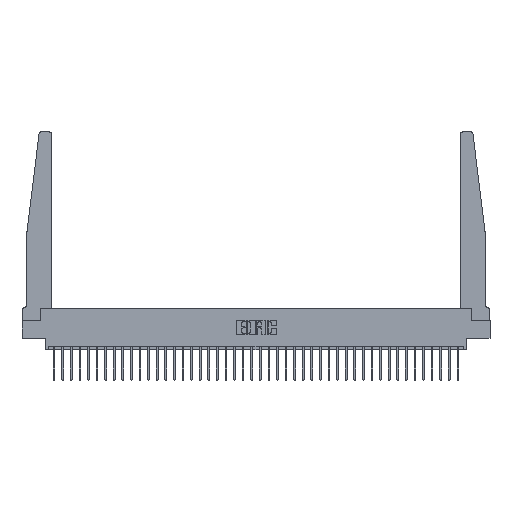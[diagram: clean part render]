
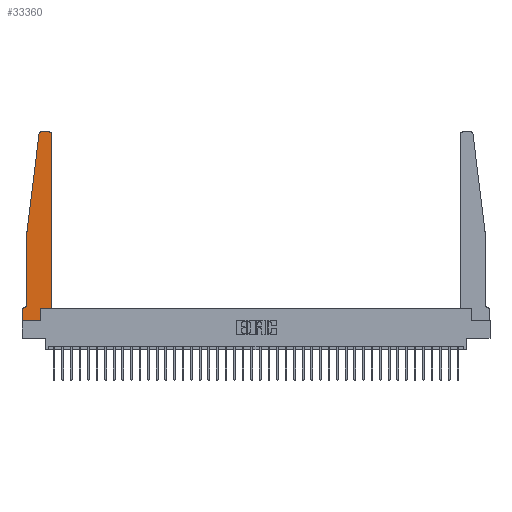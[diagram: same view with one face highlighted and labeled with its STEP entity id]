
A CAD part, top view. The second image highlights one B-rep face of the part: STEP entity #33360.
In plain terms, the highlighted planar face has unit normal (0, 0, 1).
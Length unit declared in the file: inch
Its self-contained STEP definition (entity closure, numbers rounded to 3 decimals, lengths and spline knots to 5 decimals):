
#503 = VECTOR ( 'NONE', #7519, 39.37008 ) ;
#725 = CARTESIAN_POINT ( 'NONE',  ( 0.065, 1.25, 0.37 ) ) ;
#1184 = EDGE_CURVE ( 'NONE', #20355, #28076, #22649, .T. ) ;
#1541 = DIRECTION ( 'NONE',  ( 0., 1., 0. ) ) ;
#1736 = ORIENTED_EDGE ( 'NONE', *, *, #19785, .T. ) ;
#2650 = CARTESIAN_POINT ( 'NONE',  ( 0.2605, 0., 0.37 ) ) ;
#3480 = CARTESIAN_POINT ( 'NONE',  ( 0.2605, 0.18, 0.37 ) ) ;
#3515 = ORIENTED_EDGE ( 'NONE', *, *, #10122, .T. ) ;
#4983 = EDGE_CURVE ( 'NONE', #23676, #20355, #24032, .T. ) ;
#5235 = EDGE_LOOP ( 'NONE', ( #27498, #21151, #14736, #30048, #1736, #3515, #18180, #26234, #5268, #14332, #15177, #31348 ) ) ;
#5259 = CARTESIAN_POINT ( 'NONE',  ( 0.27653, 2.72, 0.37 ) ) ;
#5268 = ORIENTED_EDGE ( 'NONE', *, *, #14583, .T. ) ;
#5748 = VECTOR ( 'NONE', #14102, 39.37008 ) ;
#5788 = LINE ( 'NONE', #28408, #20397 ) ;
#7519 = DIRECTION ( 'NONE',  ( 1., 0., 0. ) ) ;
#8059 = DIRECTION ( 'NONE',  ( 1., 0., 0. ) ) ;
#8507 = VERTEX_POINT ( 'NONE', #22959 ) ;
#8727 = CARTESIAN_POINT ( 'NONE',  ( 0.065, 0.2375, 0.37 ) ) ;
#9334 = DIRECTION ( 'NONE',  ( -1., 0., 0. ) ) ;
#9636 = EDGE_CURVE ( 'NONE', #8507, #23676, #5788, .T. ) ;
#9638 = DIRECTION ( 'NONE',  ( 0., 0., 1. ) ) ;
#9704 = CARTESIAN_POINT ( 'NONE',  ( 0.425, 2.72, 0.37 ) ) ;
#9850 = EDGE_CURVE ( 'NONE', #31163, #11322, #15240, .T. ) ;
#9877 = LINE ( 'NONE', #23579, #30777 ) ;
#10122 = EDGE_CURVE ( 'NONE', #10125, #17348, #14800, .T. ) ;
#10125 = VERTEX_POINT ( 'NONE', #14221 ) ;
#11322 = VERTEX_POINT ( 'NONE', #2650 ) ;
#11602 = DIRECTION ( 'NONE',  ( 0., 0., -1. ) ) ;
#12517 = AXIS2_PLACEMENT_3D ( 'NONE', #27898, #11602, #30634 ) ;
#12874 = DIRECTION ( 'NONE',  ( 0., 0., 1. ) ) ;
#13683 = VECTOR ( 'NONE', #19282, 39.37008 ) ;
#13777 = CARTESIAN_POINT ( 'NONE',  ( 0.2605, 0.18, 0.37 ) ) ;
#14102 = DIRECTION ( 'NONE',  ( -1., 0., 0. ) ) ;
#14221 = CARTESIAN_POINT ( 'NONE',  ( 0.015, 0.1875, 0.37 ) ) ;
#14332 = ORIENTED_EDGE ( 'NONE', *, *, #14438, .T. ) ;
#14438 = EDGE_CURVE ( 'NONE', #29267, #26822, #21063, .T. ) ;
#14583 = EDGE_CURVE ( 'NONE', #11322, #29267, #16778, .T. ) ;
#14736 = ORIENTED_EDGE ( 'NONE', *, *, #1184, .T. ) ;
#14800 = LINE ( 'NONE', #19615, #5748 ) ;
#15177 = ORIENTED_EDGE ( 'NONE', *, *, #20769, .T. ) ;
#15240 = LINE ( 'NONE', #23872, #503 ) ;
#16525 = DIRECTION ( 'NONE',  ( 0., 1., 0. ) ) ;
#16778 = LINE ( 'NONE', #13777, #30385 ) ;
#17348 = VERTEX_POINT ( 'NONE', #24806 ) ;
#17483 = LINE ( 'NONE', #34317, #31080 ) ;
#18180 = ORIENTED_EDGE ( 'NONE', *, *, #28186, .T. ) ;
#18365 = EDGE_CURVE ( 'NONE', #28076, #25143, #18479, .T. ) ;
#18479 = LINE ( 'NONE', #21705, #32872 ) ;
#19282 = DIRECTION ( 'NONE',  ( -0.122, -0.992, 0. ) ) ;
#19615 = CARTESIAN_POINT ( 'NONE',  ( 0.065, 0.1875, 0.37 ) ) ;
#19785 = EDGE_CURVE ( 'NONE', #25143, #10125, #33612, .T. ) ;
#20355 = VERTEX_POINT ( 'NONE', #24633 ) ;
#20397 = VECTOR ( 'NONE', #9334, 39.37008 ) ;
#20769 = EDGE_CURVE ( 'NONE', #26822, #28804, #17483, .T. ) ;
#21063 = LINE ( 'NONE', #21426, #34589 ) ;
#21151 = ORIENTED_EDGE ( 'NONE', *, *, #4983, .T. ) ;
#21426 = CARTESIAN_POINT ( 'NONE',  ( 0.425, 0.18, 0.37 ) ) ;
#21705 = CARTESIAN_POINT ( 'NONE',  ( 0.065, 1.25, 0.37 ) ) ;
#22135 = CARTESIAN_POINT ( 'NONE',  ( 0.425, 0.18, 0.37 ) ) ;
#22649 = LINE ( 'NONE', #30055, #13683 ) ;
#22959 = CARTESIAN_POINT ( 'NONE',  ( 0.395, 2.75, 0.37 ) ) ;
#23236 = PLANE ( 'NONE',  #24862 ) ;
#23579 = CARTESIAN_POINT ( 'NONE',  ( 0., 0., 0.37 ) ) ;
#23676 = VERTEX_POINT ( 'NONE', #24871 ) ;
#23872 = CARTESIAN_POINT ( 'NONE',  ( 0., 0., 0.37 ) ) ;
#24032 = CIRCLE ( 'NONE', #32493, 0.03 ) ;
#24122 = DIRECTION ( 'NONE',  ( 1., 0., 0. ) ) ;
#24399 = DIRECTION ( 'NONE',  ( 0., 0., 1. ) ) ;
#24633 = CARTESIAN_POINT ( 'NONE',  ( 0.24675, 2.72367, 0.37 ) ) ;
#24806 = CARTESIAN_POINT ( 'NONE',  ( 0., 0.1875, 0.37 ) ) ;
#24862 = AXIS2_PLACEMENT_3D ( 'NONE', #25980, #9638, #28718 ) ;
#24871 = CARTESIAN_POINT ( 'NONE',  ( 0.27653, 2.75, 0.37 ) ) ;
#25143 = VERTEX_POINT ( 'NONE', #8727 ) ;
#25271 = AXIS2_PLACEMENT_3D ( 'NONE', #29167, #12874, #31894 ) ;
#25485 = FACE_OUTER_BOUND ( 'NONE', #5235, .T. ) ;
#25524 = CARTESIAN_POINT ( 'NONE',  ( 0., 0., 0.37 ) ) ;
#25980 = CARTESIAN_POINT ( 'NONE',  ( 0., 0.1875, 0.37 ) ) ;
#26234 = ORIENTED_EDGE ( 'NONE', *, *, #9850, .T. ) ;
#26321 = DIRECTION ( 'NONE',  ( 0., -1., 0. ) ) ;
#26822 = VERTEX_POINT ( 'NONE', #22135 ) ;
#27498 = ORIENTED_EDGE ( 'NONE', *, *, #9636, .T. ) ;
#27898 = CARTESIAN_POINT ( 'NONE',  ( 0.015, 0.2375, 0.37 ) ) ;
#28076 = VERTEX_POINT ( 'NONE', #725 ) ;
#28186 = EDGE_CURVE ( 'NONE', #17348, #31163, #9877, .T. ) ;
#28408 = CARTESIAN_POINT ( 'NONE',  ( 0.25, 2.75, 0.37 ) ) ;
#28718 = DIRECTION ( 'NONE',  ( 1., 0., 0. ) ) ;
#28804 = VERTEX_POINT ( 'NONE', #9704 ) ;
#29167 = CARTESIAN_POINT ( 'NONE',  ( 0.395, 2.72, 0.37 ) ) ;
#29267 = VERTEX_POINT ( 'NONE', #3480 ) ;
#30048 = ORIENTED_EDGE ( 'NONE', *, *, #18365, .T. ) ;
#30055 = CARTESIAN_POINT ( 'NONE',  ( 0.065, 1.25, 0.37 ) ) ;
#30276 = CIRCLE ( 'NONE', #25271, 0.03 ) ;
#30385 = VECTOR ( 'NONE', #16525, 39.37008 ) ;
#30634 = DIRECTION ( 'NONE',  ( -1., 0., 0. ) ) ;
#30777 = VECTOR ( 'NONE', #26321, 39.37008 ) ;
#31080 = VECTOR ( 'NONE', #1541, 39.37008 ) ;
#31163 = VERTEX_POINT ( 'NONE', #25524 ) ;
#31348 = ORIENTED_EDGE ( 'NONE', *, *, #32025, .T. ) ;
#31894 = DIRECTION ( 'NONE',  ( 1., 0., 0. ) ) ;
#32025 = EDGE_CURVE ( 'NONE', #28804, #8507, #30276, .T. ) ;
#32493 = AXIS2_PLACEMENT_3D ( 'NONE', #5259, #24399, #8059 ) ;
#32872 = VECTOR ( 'NONE', #35156, 39.37008 ) ;
#33360 = ADVANCED_FACE ( 'NONE', ( #25485 ), #23236, .T. ) ;
#33612 = CIRCLE ( 'NONE', #12517, 0.05 ) ;
#34317 = CARTESIAN_POINT ( 'NONE',  ( 0.425, 0.18, 0.37 ) ) ;
#34589 = VECTOR ( 'NONE', #24122, 39.37008 ) ;
#35156 = DIRECTION ( 'NONE',  ( 0., -1., 0. ) ) ;
